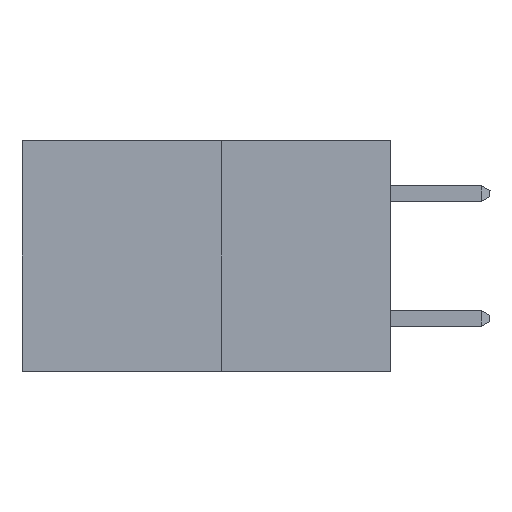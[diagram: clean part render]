
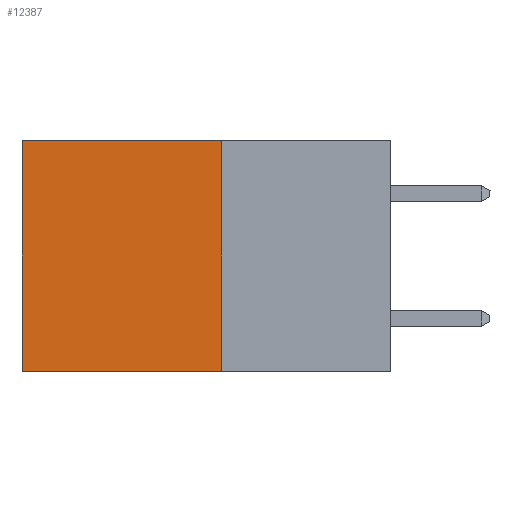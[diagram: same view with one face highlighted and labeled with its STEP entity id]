
A CAD part, left-side view. The second image highlights one B-rep face of the part: STEP entity #12387.
In plain terms, the highlighted planar face has unit normal (-1, 0, 0).
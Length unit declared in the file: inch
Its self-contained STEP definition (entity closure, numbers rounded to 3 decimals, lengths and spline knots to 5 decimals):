
#194 = VECTOR ( 'NONE', #10999, 39.37008 ) ;
#470 = LINE ( 'NONE', #14281, #2847 ) ;
#622 = EDGE_CURVE ( 'NONE', #11882, #3281, #470, .T. ) ;
#761 = CARTESIAN_POINT ( 'NONE',  ( 0.277, 0.59, -0.37 ) ) ;
#855 = ORIENTED_EDGE ( 'NONE', *, *, #14217, .F. ) ;
#1656 = VECTOR ( 'NONE', #6526, 39.37008 ) ;
#2338 = ORIENTED_EDGE ( 'NONE', *, *, #622, .F. ) ;
#2847 = VECTOR ( 'NONE', #9567, 39.37008 ) ;
#3249 = VECTOR ( 'NONE', #3320, 39.37008 ) ;
#3281 = VERTEX_POINT ( 'NONE', #761 ) ;
#3320 = DIRECTION ( 'NONE',  ( 0., 0., -1. ) ) ;
#3551 = VERTEX_POINT ( 'NONE', #8610 ) ;
#5355 = DIRECTION ( 'NONE',  ( 1., 0., 0. ) ) ;
#6260 = FACE_OUTER_BOUND ( 'NONE', #14680, .T. ) ;
#6489 = VERTEX_POINT ( 'NONE', #7911 ) ;
#6526 = DIRECTION ( 'NONE',  ( 0., 0., -1. ) ) ;
#6808 = LINE ( 'NONE', #13308, #194 ) ;
#7510 = ORIENTED_EDGE ( 'NONE', *, *, #13478, .T. ) ;
#7765 = CARTESIAN_POINT ( 'NONE',  ( 0.277, 0.27, -0.37 ) ) ;
#7911 = CARTESIAN_POINT ( 'NONE',  ( 0.277, 0.27, 0. ) ) ;
#8610 = CARTESIAN_POINT ( 'NONE',  ( 0.277, 0.59, 0. ) ) ;
#9567 = DIRECTION ( 'NONE',  ( 0., 1., 0. ) ) ;
#10145 = CARTESIAN_POINT ( 'NONE',  ( 0.277, 0.27, -0.37 ) ) ;
#10999 = DIRECTION ( 'NONE',  ( 0., 1., 0. ) ) ;
#11088 = LINE ( 'NONE', #7765, #1656 ) ;
#11198 = AXIS2_PLACEMENT_3D ( 'NONE', #10145, #5355, #13705 ) ;
#11353 = PLANE ( 'NONE',  #11198 ) ;
#11882 = VERTEX_POINT ( 'NONE', #14563 ) ;
#12379 = LINE ( 'NONE', #12776, #3249 ) ;
#12387 = ADVANCED_FACE ( 'NONE', ( #6260 ), #11353, .F. ) ;
#12776 = CARTESIAN_POINT ( 'NONE',  ( 0.277, 0.59, -0.37 ) ) ;
#13308 = CARTESIAN_POINT ( 'NONE',  ( 0.277, 0.27, 0. ) ) ;
#13478 = EDGE_CURVE ( 'NONE', #6489, #3551, #6808, .T. ) ;
#13705 = DIRECTION ( 'NONE',  ( 0., 0., -1. ) ) ;
#13967 = ORIENTED_EDGE ( 'NONE', *, *, #15237, .T. ) ;
#14217 = EDGE_CURVE ( 'NONE', #6489, #11882, #11088, .T. ) ;
#14281 = CARTESIAN_POINT ( 'NONE',  ( 0.277, 0.27, -0.37 ) ) ;
#14563 = CARTESIAN_POINT ( 'NONE',  ( 0.277, 0.27, -0.37 ) ) ;
#14680 = EDGE_LOOP ( 'NONE', ( #13967, #2338, #855, #7510 ) ) ;
#15237 = EDGE_CURVE ( 'NONE', #3551, #3281, #12379, .T. ) ;
